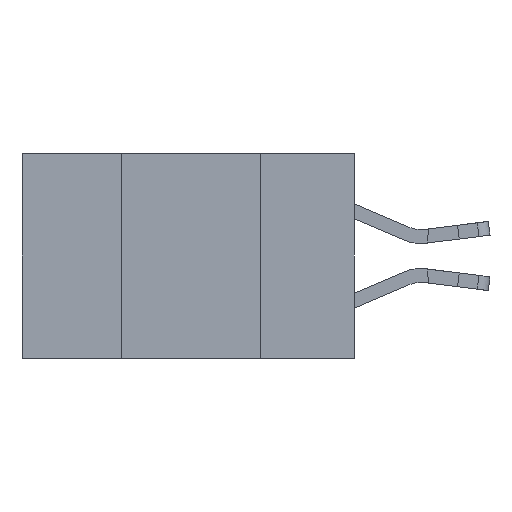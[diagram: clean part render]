
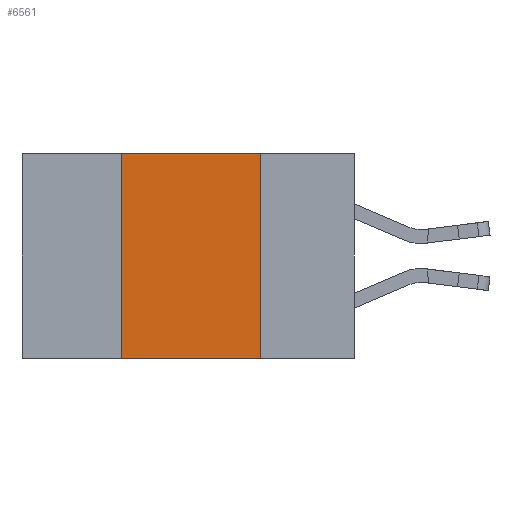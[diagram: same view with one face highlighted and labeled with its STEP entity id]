
A CAD part, left-side view. The second image highlights one B-rep face of the part: STEP entity #6561.
In plain terms, the highlighted planar face has unit normal (-1, 0, 0).
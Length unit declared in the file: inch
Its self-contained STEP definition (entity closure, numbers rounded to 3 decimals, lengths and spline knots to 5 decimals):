
#603 = DIRECTION ( 'NONE',  ( 0., 0., 1. ) ) ;
#889 = FACE_OUTER_BOUND ( 'NONE', #7978, .T. ) ;
#1139 = VERTEX_POINT ( 'NONE', #18037 ) ;
#1155 = DIRECTION ( 'NONE',  ( 0., 0., -1. ) ) ;
#1391 = VERTEX_POINT ( 'NONE', #8346 ) ;
#2157 = CARTESIAN_POINT ( 'NONE',  ( 0., 0.6, -0.37 ) ) ;
#2589 = LINE ( 'NONE', #14280, #8867 ) ;
#3385 = CARTESIAN_POINT ( 'NONE',  ( 0., 0.6, 0. ) ) ;
#3573 = VERTEX_POINT ( 'NONE', #5013 ) ;
#4466 = VERTEX_POINT ( 'NONE', #11434 ) ;
#5013 = CARTESIAN_POINT ( 'NONE',  ( 0., 0.42, 0. ) ) ;
#5772 = VECTOR ( 'NONE', #13987, 39.37008 ) ;
#5904 = ORIENTED_EDGE ( 'NONE', *, *, #17899, .F. ) ;
#6561 = ADVANCED_FACE ( 'NONE', ( #889 ), #8272, .F. ) ;
#6745 = DIRECTION ( 'NONE',  ( 1., 0., 0. ) ) ;
#6780 = VECTOR ( 'NONE', #603, 39.37008 ) ;
#7978 = EDGE_LOOP ( 'NONE', ( #16472, #5904, #8256, #10448 ) ) ;
#8089 = DIRECTION ( 'NONE',  ( 0., 0., -1. ) ) ;
#8256 = ORIENTED_EDGE ( 'NONE', *, *, #14627, .F. ) ;
#8272 = PLANE ( 'NONE',  #15422 ) ;
#8346 = CARTESIAN_POINT ( 'NONE',  ( 0., 0.42, -0.37 ) ) ;
#8867 = VECTOR ( 'NONE', #1155, 39.37008 ) ;
#10448 = ORIENTED_EDGE ( 'NONE', *, *, #11954, .T. ) ;
#11207 = EDGE_CURVE ( 'NONE', #1139, #4466, #2589, .T. ) ;
#11238 = LINE ( 'NONE', #2157, #15565 ) ;
#11434 = CARTESIAN_POINT ( 'NONE',  ( 0., 0.17, -0.37 ) ) ;
#11954 = EDGE_CURVE ( 'NONE', #1391, #4466, #11238, .T. ) ;
#12201 = CARTESIAN_POINT ( 'NONE',  ( 0., 0.42, -0.37 ) ) ;
#12462 = LINE ( 'NONE', #3385, #5772 ) ;
#13987 = DIRECTION ( 'NONE',  ( 0., -1., 0. ) ) ;
#14014 = DIRECTION ( 'NONE',  ( 0., -1., 0. ) ) ;
#14280 = CARTESIAN_POINT ( 'NONE',  ( 0., 0.17, -0.37 ) ) ;
#14627 = EDGE_CURVE ( 'NONE', #1391, #3573, #18420, .T. ) ;
#15422 = AXIS2_PLACEMENT_3D ( 'NONE', #18516, #6745, #8089 ) ;
#15565 = VECTOR ( 'NONE', #14014, 39.37008 ) ;
#16472 = ORIENTED_EDGE ( 'NONE', *, *, #11207, .F. ) ;
#17899 = EDGE_CURVE ( 'NONE', #3573, #1139, #12462, .T. ) ;
#18037 = CARTESIAN_POINT ( 'NONE',  ( 0., 0.17, 0. ) ) ;
#18420 = LINE ( 'NONE', #12201, #6780 ) ;
#18516 = CARTESIAN_POINT ( 'NONE',  ( 0., 0.6, 0. ) ) ;
